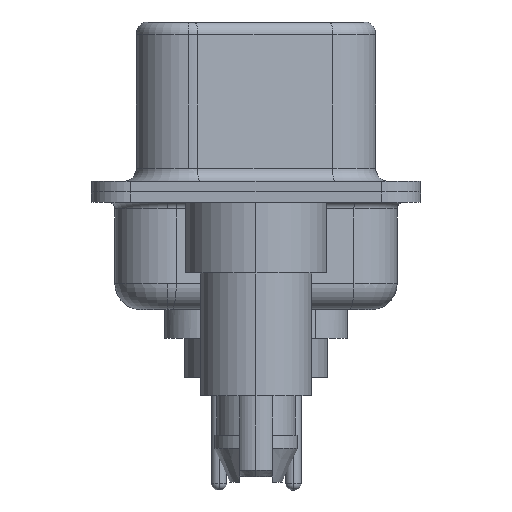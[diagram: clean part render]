
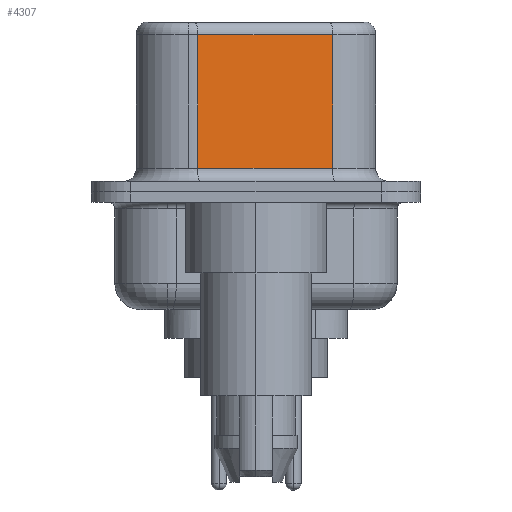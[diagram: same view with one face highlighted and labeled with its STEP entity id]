
A CAD part, left-side view. The second image highlights one B-rep face of the part: STEP entity #4307.
In plain terms, the highlighted planar face has unit normal (-0.985, -0.174, 0).
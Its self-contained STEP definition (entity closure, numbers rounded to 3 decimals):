
#782 = LINE ( 'NONE', #20001, #9197 ) ;
#833 = DIRECTION ( 'NONE',  ( 0.985, 0.174, 0. ) ) ;
#866 = ORIENTED_EDGE ( 'NONE', *, *, #12473, .F. ) ;
#1851 = VERTEX_POINT ( 'NONE', #17844 ) ;
#2048 = DIRECTION ( 'NONE',  ( 0., 0., -1. ) ) ;
#2680 = DIRECTION ( 'NONE',  ( -0.174, 0.985, 0. ) ) ;
#3135 = CARTESIAN_POINT ( 'NONE',  ( 4.585, -2.927, 6.02 ) ) ;
#3307 = EDGE_LOOP ( 'NONE', ( #866, #8128, #10161, #21429 ) ) ;
#4307 = ADVANCED_FACE ( 'NONE', ( #13231 ), #13010, .F. ) ;
#5647 = CARTESIAN_POINT ( 'NONE',  ( 3.675, 2.233, 6.52 ) ) ;
#6104 = DIRECTION ( 'NONE',  ( 0., 0., -1. ) ) ;
#6574 = LINE ( 'NONE', #18754, #10282 ) ;
#7347 = DIRECTION ( 'NONE',  ( -0.174, 0.985, 0. ) ) ;
#8128 = ORIENTED_EDGE ( 'NONE', *, *, #10779, .T. ) ;
#9119 = DIRECTION ( 'NONE',  ( 0.174, -0.985, 0. ) ) ;
#9197 = VECTOR ( 'NONE', #7347, 1000. ) ;
#10161 = ORIENTED_EDGE ( 'NONE', *, *, #21022, .T. ) ;
#10282 = VECTOR ( 'NONE', #6104, 1000. ) ;
#10779 = EDGE_CURVE ( 'NONE', #13214, #22547, #782, .T. ) ;
#11492 = CARTESIAN_POINT ( 'NONE',  ( 4.585, -2.927, 6.52 ) ) ;
#11703 = CARTESIAN_POINT ( 'NONE',  ( 3.675, 2.233, 0.9 ) ) ;
#12209 = EDGE_CURVE ( 'NONE', #14418, #1851, #19597, .T. ) ;
#12473 = EDGE_CURVE ( 'NONE', #13214, #1851, #6574, .T. ) ;
#12780 = LINE ( 'NONE', #5647, #17002 ) ;
#13010 = PLANE ( 'NONE',  #22873 ) ;
#13214 = VERTEX_POINT ( 'NONE', #3135 ) ;
#13231 = FACE_OUTER_BOUND ( 'NONE', #3307, .T. ) ;
#14418 = VERTEX_POINT ( 'NONE', #11703 ) ;
#14782 = VECTOR ( 'NONE', #9119, 1000. ) ;
#15877 = CARTESIAN_POINT ( 'NONE',  ( 3.675, 2.233, 6.02 ) ) ;
#17002 = VECTOR ( 'NONE', #2048, 1000. ) ;
#17844 = CARTESIAN_POINT ( 'NONE',  ( 4.585, -2.927, 0.9 ) ) ;
#18754 = CARTESIAN_POINT ( 'NONE',  ( 4.585, -2.927, 6.52 ) ) ;
#19597 = LINE ( 'NONE', #19943, #14782 ) ;
#19943 = CARTESIAN_POINT ( 'NONE',  ( 4.585, -2.927, 0.9 ) ) ;
#20001 = CARTESIAN_POINT ( 'NONE',  ( 4.585, -2.927, 6.02 ) ) ;
#21022 = EDGE_CURVE ( 'NONE', #22547, #14418, #12780, .T. ) ;
#21429 = ORIENTED_EDGE ( 'NONE', *, *, #12209, .T. ) ;
#22547 = VERTEX_POINT ( 'NONE', #15877 ) ;
#22873 = AXIS2_PLACEMENT_3D ( 'NONE', #11492, #833, #2680 ) ;
